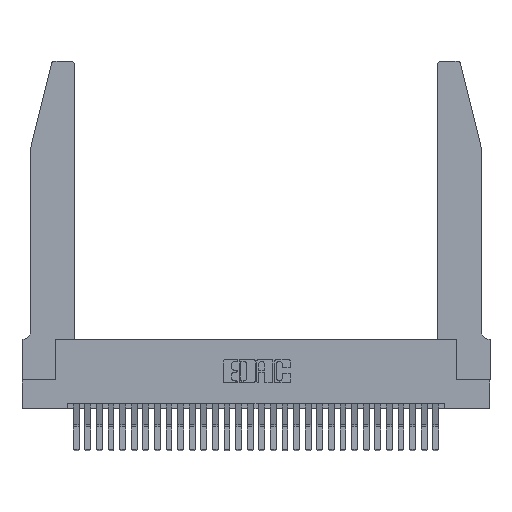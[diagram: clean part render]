
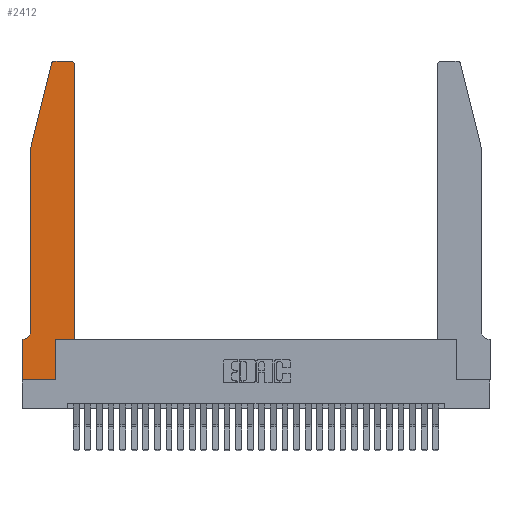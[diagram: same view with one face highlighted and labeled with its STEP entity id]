
A CAD part, top view. The second image highlights one B-rep face of the part: STEP entity #2412.
In plain terms, the highlighted planar face has unit normal (0, 0, 1).
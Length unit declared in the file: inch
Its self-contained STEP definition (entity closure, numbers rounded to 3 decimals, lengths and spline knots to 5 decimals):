
#583 = CARTESIAN_POINT ( 'NONE',  ( 0.284, 2.75, 0.37 ) ) ;
#727 = CARTESIAN_POINT ( 'NONE',  ( 0.0755, 0.35, 0.37 ) ) ;
#967 = LINE ( 'NONE', #727, #26820 ) ;
#1128 = AXIS2_PLACEMENT_3D ( 'NONE', #13819, #30380, #16215 ) ;
#1174 = CARTESIAN_POINT ( 'NONE',  ( 0.4205, 2.75, 0.37 ) ) ;
#1431 = CARTESIAN_POINT ( 'NONE',  ( 0.4505, 0.35, 0.37 ) ) ;
#2111 = EDGE_CURVE ( 'NONE', #9526, #2267, #19772, .T. ) ;
#2267 = VERTEX_POINT ( 'NONE', #8569 ) ;
#2274 = CARTESIAN_POINT ( 'NONE',  ( 0.4505, 2.72, 0.37 ) ) ;
#2412 = ADVANCED_FACE ( 'NONE', ( #12306 ), #6574, .T. ) ;
#2570 = CARTESIAN_POINT ( 'NONE',  ( 0.4505, 0.35, 0.37 ) ) ;
#2843 = EDGE_CURVE ( 'NONE', #7640, #11863, #967, .T. ) ;
#2962 = CARTESIAN_POINT ( 'NONE',  ( 0.2865, 0.35, 0.37 ) ) ;
#3088 = ORIENTED_EDGE ( 'NONE', *, *, #10516, .T. ) ;
#3365 = CARTESIAN_POINT ( 'NONE',  ( 0.4205, 2.72, 0.37 ) ) ;
#3524 = DIRECTION ( 'NONE',  ( 0., -1., 0. ) ) ;
#3623 = EDGE_CURVE ( 'NONE', #7018, #29006, #6812, .T. ) ;
#4287 = CIRCLE ( 'NONE', #19154, 0.03 ) ;
#4332 = EDGE_CURVE ( 'NONE', #12272, #27269, #19314, .T. ) ;
#4696 = ORIENTED_EDGE ( 'NONE', *, *, #26404, .T. ) ;
#4959 = CARTESIAN_POINT ( 'NONE',  ( 0.2865, 0., 0.37 ) ) ;
#5901 = DIRECTION ( 'NONE',  ( 1., 0., 0. ) ) ;
#6418 = VECTOR ( 'NONE', #19613, 39.37008 ) ;
#6574 = PLANE ( 'NONE',  #7533 ) ;
#6668 = CARTESIAN_POINT ( 'NONE',  ( 0.2605, 2.75, 0.37 ) ) ;
#6812 = LINE ( 'NONE', #20740, #18226 ) ;
#7018 = VERTEX_POINT ( 'NONE', #15591 ) ;
#7453 = ORIENTED_EDGE ( 'NONE', *, *, #18317, .T. ) ;
#7533 = AXIS2_PLACEMENT_3D ( 'NONE', #23477, #25852, #11609 ) ;
#7584 = DIRECTION ( 'NONE',  ( 1., 0., 0. ) ) ;
#7640 = VERTEX_POINT ( 'NONE', #26882 ) ;
#8091 = VECTOR ( 'NONE', #25955, 39.37008 ) ;
#8467 = CARTESIAN_POINT ( 'NONE',  ( 0.0055, 0.42, 0.37 ) ) ;
#8498 = DIRECTION ( 'NONE',  ( -0.239, -0.971, 0. ) ) ;
#8569 = CARTESIAN_POINT ( 'NONE',  ( 0.2865, 0.35, 0.37 ) ) ;
#9526 = VERTEX_POINT ( 'NONE', #4959 ) ;
#10516 = EDGE_CURVE ( 'NONE', #22109, #7018, #25806, .T. ) ;
#10541 = DIRECTION ( 'NONE',  ( 0., 1., 0. ) ) ;
#10971 = DIRECTION ( 'NONE',  ( -1., 0., 0. ) ) ;
#11003 = CARTESIAN_POINT ( 'NONE',  ( 0.0755, 2., 0.37 ) ) ;
#11355 = EDGE_CURVE ( 'NONE', #22976, #12426, #14630, .T. ) ;
#11609 = DIRECTION ( 'NONE',  ( 1., 0., 0. ) ) ;
#11735 = ORIENTED_EDGE ( 'NONE', *, *, #2111, .T. ) ;
#11863 = VERTEX_POINT ( 'NONE', #22813 ) ;
#12272 = VERTEX_POINT ( 'NONE', #2570 ) ;
#12306 = FACE_OUTER_BOUND ( 'NONE', #17084, .T. ) ;
#12426 = VERTEX_POINT ( 'NONE', #583 ) ;
#12962 = VECTOR ( 'NONE', #18622, 39.37008 ) ;
#13018 = LINE ( 'NONE', #14837, #6418 ) ;
#13062 = EDGE_CURVE ( 'NONE', #12426, #22109, #26773, .T. ) ;
#13178 = VECTOR ( 'NONE', #8498, 39.37008 ) ;
#13437 = VECTOR ( 'NONE', #10541, 39.37008 ) ;
#13819 = CARTESIAN_POINT ( 'NONE',  ( 0.284, 2.72, 0.37 ) ) ;
#14630 = LINE ( 'NONE', #6668, #8091 ) ;
#14837 = CARTESIAN_POINT ( 'NONE',  ( 0., 0., 0.37 ) ) ;
#15091 = VECTOR ( 'NONE', #19817, 39.37008 ) ;
#15500 = ORIENTED_EDGE ( 'NONE', *, *, #4332, .T. ) ;
#15591 = CARTESIAN_POINT ( 'NONE',  ( 0.0755, 2., 0.37 ) ) ;
#15839 = LINE ( 'NONE', #24479, #15091 ) ;
#16215 = DIRECTION ( 'NONE',  ( 1., 0., 0. ) ) ;
#16268 = ORIENTED_EDGE ( 'NONE', *, *, #20040, .T. ) ;
#16589 = CARTESIAN_POINT ( 'NONE',  ( 0., 0., 0.37 ) ) ;
#17084 = EDGE_LOOP ( 'NONE', ( #20300, #21811, #3088, #29540, #4696, #26978, #22188, #29921, #11735, #7453, #15500, #16268 ) ) ;
#17270 = CARTESIAN_POINT ( 'NONE',  ( 0.4505, 0.35, 0.37 ) ) ;
#17494 = VERTEX_POINT ( 'NONE', #16589 ) ;
#17802 = VECTOR ( 'NONE', #7584, 39.37008 ) ;
#17952 = DIRECTION ( 'NONE',  ( -1., 0., 0. ) ) ;
#18226 = VECTOR ( 'NONE', #3524, 39.37008 ) ;
#18317 = EDGE_CURVE ( 'NONE', #2267, #12272, #30391, .T. ) ;
#18372 = CARTESIAN_POINT ( 'NONE',  ( 0.25487, 2.72718, 0.37 ) ) ;
#18622 = DIRECTION ( 'NONE',  ( 0., 1., 0. ) ) ;
#19052 = AXIS2_PLACEMENT_3D ( 'NONE', #8467, #25225, #10971 ) ;
#19154 = AXIS2_PLACEMENT_3D ( 'NONE', #3365, #20470, #5901 ) ;
#19314 = LINE ( 'NONE', #1431, #12962 ) ;
#19595 = CARTESIAN_POINT ( 'NONE',  ( 0.0755, 0.42, 0.37 ) ) ;
#19613 = DIRECTION ( 'NONE',  ( 1., 0., 0. ) ) ;
#19772 = LINE ( 'NONE', #2962, #13437 ) ;
#19817 = DIRECTION ( 'NONE',  ( 0., -1., 0. ) ) ;
#20040 = EDGE_CURVE ( 'NONE', #27269, #22976, #4287, .T. ) ;
#20300 = ORIENTED_EDGE ( 'NONE', *, *, #11355, .T. ) ;
#20470 = DIRECTION ( 'NONE',  ( 0., 0., 1. ) ) ;
#20524 = EDGE_CURVE ( 'NONE', #11863, #17494, #15839, .T. ) ;
#20740 = CARTESIAN_POINT ( 'NONE',  ( 0.0755, 2., 0.37 ) ) ;
#21811 = ORIENTED_EDGE ( 'NONE', *, *, #13062, .T. ) ;
#22109 = VERTEX_POINT ( 'NONE', #18372 ) ;
#22188 = ORIENTED_EDGE ( 'NONE', *, *, #20524, .T. ) ;
#22813 = CARTESIAN_POINT ( 'NONE',  ( 0., 0.35, 0.37 ) ) ;
#22976 = VERTEX_POINT ( 'NONE', #1174 ) ;
#23477 = CARTESIAN_POINT ( 'NONE',  ( 0., 0.35, 0.37 ) ) ;
#24479 = CARTESIAN_POINT ( 'NONE',  ( 0., 0., 0.37 ) ) ;
#24510 = CIRCLE ( 'NONE', #19052, 0.07 ) ;
#25225 = DIRECTION ( 'NONE',  ( 0., 0., -1. ) ) ;
#25573 = EDGE_CURVE ( 'NONE', #17494, #9526, #13018, .T. ) ;
#25806 = LINE ( 'NONE', #11003, #13178 ) ;
#25852 = DIRECTION ( 'NONE',  ( 0., 0., 1. ) ) ;
#25955 = DIRECTION ( 'NONE',  ( -1., 0., 0. ) ) ;
#26404 = EDGE_CURVE ( 'NONE', #29006, #7640, #24510, .T. ) ;
#26773 = CIRCLE ( 'NONE', #1128, 0.03 ) ;
#26820 = VECTOR ( 'NONE', #17952, 39.37008 ) ;
#26882 = CARTESIAN_POINT ( 'NONE',  ( 0.0055, 0.35, 0.37 ) ) ;
#26978 = ORIENTED_EDGE ( 'NONE', *, *, #2843, .T. ) ;
#27269 = VERTEX_POINT ( 'NONE', #2274 ) ;
#29006 = VERTEX_POINT ( 'NONE', #19595 ) ;
#29540 = ORIENTED_EDGE ( 'NONE', *, *, #3623, .T. ) ;
#29921 = ORIENTED_EDGE ( 'NONE', *, *, #25573, .T. ) ;
#30380 = DIRECTION ( 'NONE',  ( 0., 0., 1. ) ) ;
#30391 = LINE ( 'NONE', #17270, #17802 ) ;
